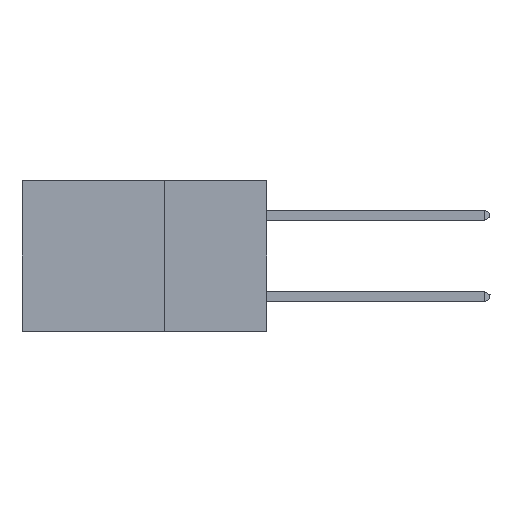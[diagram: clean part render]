
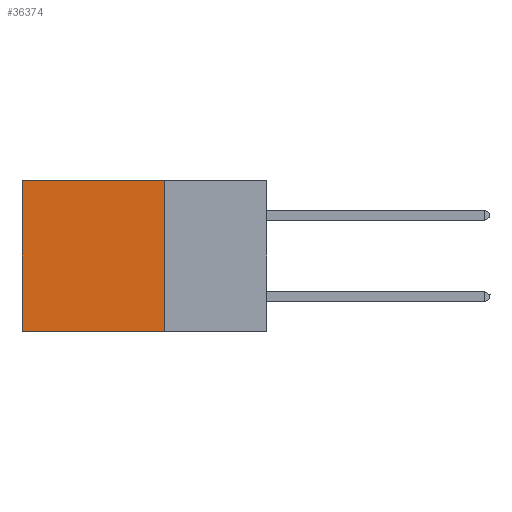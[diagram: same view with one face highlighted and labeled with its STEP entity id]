
A CAD part, left-side view. The second image highlights one B-rep face of the part: STEP entity #36374.
In plain terms, the highlighted planar face has unit normal (-1, 0, 0).
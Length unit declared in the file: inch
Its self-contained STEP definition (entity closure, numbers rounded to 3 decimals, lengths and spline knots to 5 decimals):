
#1958 = CARTESIAN_POINT ( 'NONE',  ( 0.2875, 0.25, 0. ) ) ;
#2002 = CARTESIAN_POINT ( 'NONE',  ( 0.2875, 0.6, 0. ) ) ;
#3754 = AXIS2_PLACEMENT_3D ( 'NONE', #1958, #11757, #36996 ) ;
#4344 = VECTOR ( 'NONE', #14580, 39.37008 ) ;
#4974 = CARTESIAN_POINT ( 'NONE',  ( 0.2875, 0.6, 0. ) ) ;
#5794 = VECTOR ( 'NONE', #19481, 39.37008 ) ;
#6214 = ORIENTED_EDGE ( 'NONE', *, *, #13673, .F. ) ;
#7260 = ORIENTED_EDGE ( 'NONE', *, *, #14539, .T. ) ;
#8160 = ORIENTED_EDGE ( 'NONE', *, *, #35491, .T. ) ;
#9395 = LINE ( 'NONE', #28591, #27018 ) ;
#11757 = DIRECTION ( 'NONE',  ( 1., 0., 0. ) ) ;
#13043 = CARTESIAN_POINT ( 'NONE',  ( 0.2875, 0.25, -0.37 ) ) ;
#13673 = EDGE_CURVE ( 'NONE', #30379, #28913, #38665, .T. ) ;
#14539 = EDGE_CURVE ( 'NONE', #30379, #34442, #9395, .T. ) ;
#14580 = DIRECTION ( 'NONE',  ( 0., 0., -1. ) ) ;
#15538 = EDGE_LOOP ( 'NONE', ( #8160, #21278, #6214, #7260 ) ) ;
#19469 = VECTOR ( 'NONE', #40024, 39.37008 ) ;
#19481 = DIRECTION ( 'NONE',  ( 0., 0., -1. ) ) ;
#20932 = PLANE ( 'NONE',  #3754 ) ;
#21278 = ORIENTED_EDGE ( 'NONE', *, *, #25844, .F. ) ;
#22211 = CARTESIAN_POINT ( 'NONE',  ( 0.2875, 0.25, -0.37 ) ) ;
#24079 = FACE_OUTER_BOUND ( 'NONE', #15538, .T. ) ;
#25844 = EDGE_CURVE ( 'NONE', #28913, #31498, #33555, .T. ) ;
#27018 = VECTOR ( 'NONE', #28988, 39.37008 ) ;
#28526 = CARTESIAN_POINT ( 'NONE',  ( 0.2875, 0.6, -0.37 ) ) ;
#28591 = CARTESIAN_POINT ( 'NONE',  ( 0.2875, 0.25, 0. ) ) ;
#28913 = VERTEX_POINT ( 'NONE', #13043 ) ;
#28988 = DIRECTION ( 'NONE',  ( 0., 1., 0. ) ) ;
#30379 = VERTEX_POINT ( 'NONE', #32480 ) ;
#31498 = VERTEX_POINT ( 'NONE', #28526 ) ;
#32480 = CARTESIAN_POINT ( 'NONE',  ( 0.2875, 0.25, 0. ) ) ;
#33555 = LINE ( 'NONE', #22211, #19469 ) ;
#33577 = LINE ( 'NONE', #4974, #4344 ) ;
#34442 = VERTEX_POINT ( 'NONE', #2002 ) ;
#35491 = EDGE_CURVE ( 'NONE', #34442, #31498, #33577, .T. ) ;
#36374 = ADVANCED_FACE ( 'NONE', ( #24079 ), #20932, .F. ) ;
#36996 = DIRECTION ( 'NONE',  ( 0., 0., -1. ) ) ;
#38253 = CARTESIAN_POINT ( 'NONE',  ( 0.2875, 0.25, 0. ) ) ;
#38665 = LINE ( 'NONE', #38253, #5794 ) ;
#40024 = DIRECTION ( 'NONE',  ( 0., 1., 0. ) ) ;
